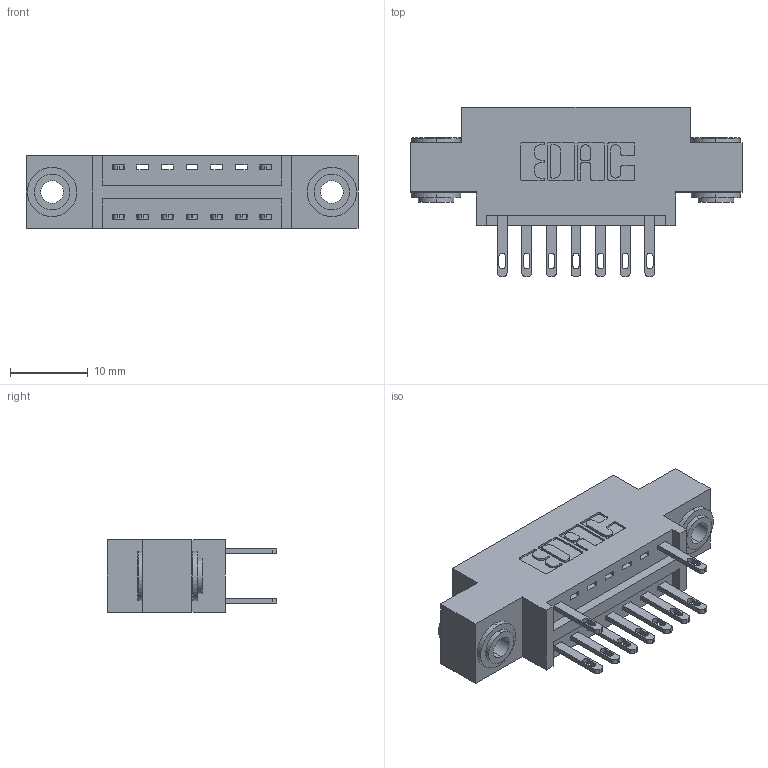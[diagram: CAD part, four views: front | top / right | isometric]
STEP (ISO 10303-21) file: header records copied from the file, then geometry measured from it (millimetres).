
FILE_DESCRIPTION (( 'STEP AP203' ), '1' );
FILE_NAME ('346-014-500-803.STEP', '2018-08-20T00:23:38', ( '' ), ( '' ), 'SwSTEP 2.0', 'SolidWorks 2016', '' );
FILE_SCHEMA (( 'CONFIG_CONTROL_DESIGN' ));
Length unit declared in the file: inch
Products named in the file (4): 346 Part_0.170 Offset - 0.156 Dia-TH; 345-292-001_345-293-100; 345-250-002_345-250-002-102; 346-014-500-803
Assembly tree (12 placements, depth 2):
  346-014-500-803
    346 Part_0.170 Offset - 0.156 Dia-TH
    345-292-001_345-293-100  x9
    345-250-002_345-250-002-102  x2
Bounding box: 42.8 x 21.84 x 9.4 mm (x, y, z)
Volume: 3748.9 mm3; surface area: 4831.5 mm2
Topology: 12 solids, 12 shells, 626 faces, 1845 edges, 1226 vertices
Faces by surface type: plane 376, cylinder 242, cone 8
Entity records: 9832 total; most frequent: CARTESIAN_POINT 1666, ORIENTED_EDGE 1598, DIRECTION 1547, EDGE_CURVE 799, VECTOR 611, LINE 611, VERTEX_POINT 530, AXIS2_PLACEMENT_3D 468
